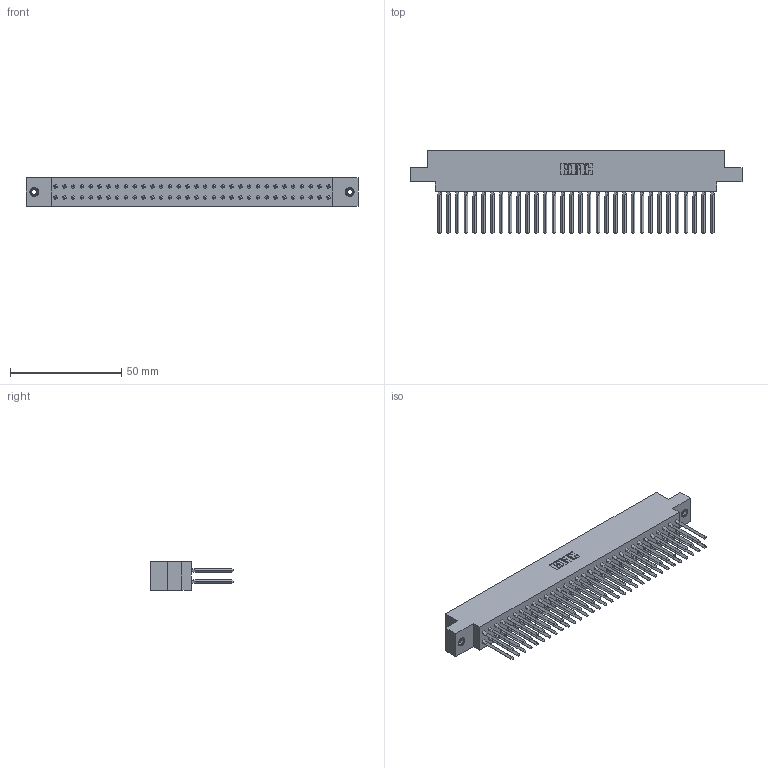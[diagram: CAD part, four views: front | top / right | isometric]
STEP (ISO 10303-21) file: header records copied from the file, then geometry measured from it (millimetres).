
FILE_DESCRIPTION (( 'STEP AP203' ), '1' );
FILE_NAME ('317-064-540-878.STEP', '2020-02-28T05:49:46', ( '' ), ( '' ), 'SwSTEP 2.0', 'SolidWorks 2016', '' );
FILE_SCHEMA (( 'CONFIG_CONTROL_DESIGN' ));
Length unit declared in the file: inch
Products named in the file (4): 317-064-540-878; 317 Part_.156 Dia - TI; 317-290-001_540; 345-250-001_345-250-003-102
Assembly tree (67 placements, depth 2):
  317-064-540-878
    317 Part_.156 Dia - TI
    317-290-001_540  x64
    345-250-001_345-250-003-102  x2
Bounding box: 149.5 x 37.34 x 12.7 mm (x, y, z)
Volume: 24746.9 mm3; surface area: 36539.9 mm2
Topology: 67 solids, 67 shells, 5858 faces, 16219 edges, 10442 vertices
Faces by surface type: plane 4762, cylinder 824, bspline 256, cone 12, torus 4
Entity records: 48837 total; most frequent: CARTESIAN_POINT 8906, ORIENTED_EDGE 8398, DIRECTION 7047, EDGE_CURVE 4199, VECTOR 3923, LINE 3923, VERTEX_POINT 2789, AXIS2_PLACEMENT_3D 1562
